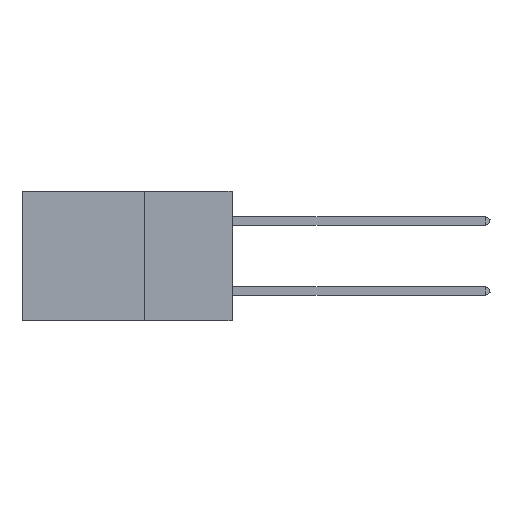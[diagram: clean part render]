
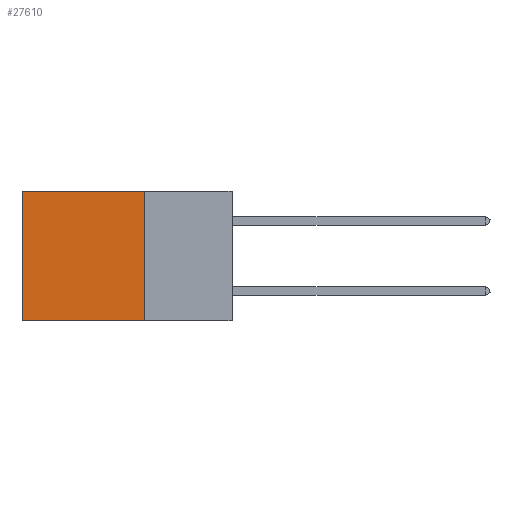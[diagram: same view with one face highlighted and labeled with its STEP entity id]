
A CAD part, left-side view. The second image highlights one B-rep face of the part: STEP entity #27610.
In plain terms, the highlighted planar face has unit normal (-1, 0, 0).
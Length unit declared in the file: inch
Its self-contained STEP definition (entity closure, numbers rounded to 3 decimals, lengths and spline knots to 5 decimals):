
#1784 = DIRECTION ( 'NONE',  ( 0., 0., -1. ) ) ;
#2111 = ORIENTED_EDGE ( 'NONE', *, *, #23049, .T. ) ;
#3067 = VERTEX_POINT ( 'NONE', #29714 ) ;
#5304 = CARTESIAN_POINT ( 'NONE',  ( 0.2875, 0.6, 0. ) ) ;
#7719 = CARTESIAN_POINT ( 'NONE',  ( 0.2875, 0.25, 0. ) ) ;
#9268 = ORIENTED_EDGE ( 'NONE', *, *, #17548, .F. ) ;
#10757 = CARTESIAN_POINT ( 'NONE',  ( 0.2875, 0.6, 0. ) ) ;
#10870 = DIRECTION ( 'NONE',  ( 0., 0., -1. ) ) ;
#11257 = CARTESIAN_POINT ( 'NONE',  ( 0.2875, 0.25, -0.37 ) ) ;
#12437 = CARTESIAN_POINT ( 'NONE',  ( 0.2875, 0.25, 0. ) ) ;
#13108 = DIRECTION ( 'NONE',  ( 0., 0., -1. ) ) ;
#13305 = CARTESIAN_POINT ( 'NONE',  ( 0.2875, 0.25, -0.37 ) ) ;
#13938 = DIRECTION ( 'NONE',  ( 0., 1., 0. ) ) ;
#14784 = EDGE_CURVE ( 'NONE', #24909, #32092, #31569, .T. ) ;
#15094 = DIRECTION ( 'NONE',  ( 0., 1., 0. ) ) ;
#16681 = EDGE_LOOP ( 'NONE', ( #19275, #9268, #22799, #2111 ) ) ;
#16865 = LINE ( 'NONE', #18075, #31073 ) ;
#17339 = VECTOR ( 'NONE', #10870, 39.37008 ) ;
#17548 = EDGE_CURVE ( 'NONE', #24115, #32092, #29536, .T. ) ;
#18075 = CARTESIAN_POINT ( 'NONE',  ( 0.2875, 0.25, 0. ) ) ;
#18891 = VECTOR ( 'NONE', #15094, 39.37008 ) ;
#19275 = ORIENTED_EDGE ( 'NONE', *, *, #14784, .T. ) ;
#19865 = EDGE_CURVE ( 'NONE', #3067, #24115, #16865, .T. ) ;
#21545 = VECTOR ( 'NONE', #13938, 39.37008 ) ;
#21659 = CARTESIAN_POINT ( 'NONE',  ( 0.2875, 0.6, -0.37 ) ) ;
#22799 = ORIENTED_EDGE ( 'NONE', *, *, #19865, .F. ) ;
#23049 = EDGE_CURVE ( 'NONE', #3067, #24909, #33097, .T. ) ;
#23098 = FACE_OUTER_BOUND ( 'NONE', #16681, .T. ) ;
#24115 = VERTEX_POINT ( 'NONE', #13305 ) ;
#24909 = VERTEX_POINT ( 'NONE', #5304 ) ;
#26399 = PLANE ( 'NONE',  #32823 ) ;
#27610 = ADVANCED_FACE ( 'NONE', ( #23098 ), #26399, .F. ) ;
#29097 = DIRECTION ( 'NONE',  ( 1., 0., 0. ) ) ;
#29536 = LINE ( 'NONE', #11257, #21545 ) ;
#29714 = CARTESIAN_POINT ( 'NONE',  ( 0.2875, 0.25, 0. ) ) ;
#31073 = VECTOR ( 'NONE', #1784, 39.37008 ) ;
#31569 = LINE ( 'NONE', #10757, #17339 ) ;
#32092 = VERTEX_POINT ( 'NONE', #21659 ) ;
#32823 = AXIS2_PLACEMENT_3D ( 'NONE', #7719, #29097, #13108 ) ;
#33097 = LINE ( 'NONE', #12437, #18891 ) ;
